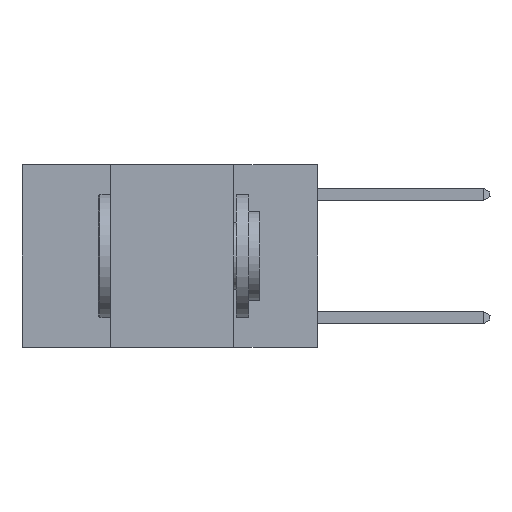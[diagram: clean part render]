
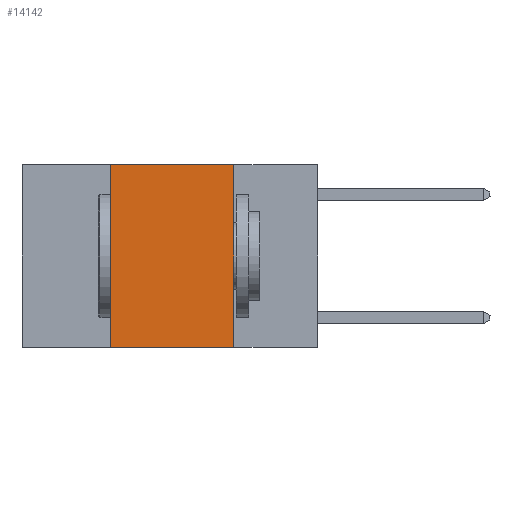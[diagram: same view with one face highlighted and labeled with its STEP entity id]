
A CAD part, left-side view. The second image highlights one B-rep face of the part: STEP entity #14142.
In plain terms, the highlighted planar face has unit normal (-1, 0, 0).
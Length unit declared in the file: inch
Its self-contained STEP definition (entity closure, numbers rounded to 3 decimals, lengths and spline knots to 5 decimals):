
#490 = CARTESIAN_POINT ( 'NONE',  ( 0., 0.42, 0. ) ) ;
#889 = VERTEX_POINT ( 'NONE', #3134 ) ;
#1014 = DIRECTION ( 'NONE',  ( 0., 0., -1. ) ) ;
#1304 = AXIS2_PLACEMENT_3D ( 'NONE', #6253, #11634, #16788 ) ;
#2366 = VECTOR ( 'NONE', #3803, 39.37008 ) ;
#2592 = CARTESIAN_POINT ( 'NONE',  ( 0., 0.17, -0.37 ) ) ;
#3063 = EDGE_CURVE ( 'NONE', #889, #5286, #8931, .T. ) ;
#3134 = CARTESIAN_POINT ( 'NONE',  ( 0., 0.42, -0.37 ) ) ;
#3528 = FACE_OUTER_BOUND ( 'NONE', #11966, .T. ) ;
#3563 = EDGE_CURVE ( 'NONE', #17010, #5286, #16999, .T. ) ;
#3803 = DIRECTION ( 'NONE',  ( 0., 0., 1. ) ) ;
#4730 = ORIENTED_EDGE ( 'NONE', *, *, #12457, .F. ) ;
#5286 = VERTEX_POINT ( 'NONE', #2592 ) ;
#6253 = CARTESIAN_POINT ( 'NONE',  ( 0., 0.6, 0. ) ) ;
#6334 = PLANE ( 'NONE',  #1304 ) ;
#7236 = CARTESIAN_POINT ( 'NONE',  ( 0., 0.6, 0. ) ) ;
#8492 = ORIENTED_EDGE ( 'NONE', *, *, #3563, .F. ) ;
#8548 = VECTOR ( 'NONE', #1014, 39.37008 ) ;
#8577 = ORIENTED_EDGE ( 'NONE', *, *, #12518, .F. ) ;
#8809 = VECTOR ( 'NONE', #13661, 39.37008 ) ;
#8931 = LINE ( 'NONE', #14211, #15452 ) ;
#11486 = LINE ( 'NONE', #16720, #2366 ) ;
#11634 = DIRECTION ( 'NONE',  ( 1., 0., 0. ) ) ;
#11966 = EDGE_LOOP ( 'NONE', ( #8492, #4730, #8577, #14532 ) ) ;
#12457 = EDGE_CURVE ( 'NONE', #17189, #17010, #16284, .T. ) ;
#12518 = EDGE_CURVE ( 'NONE', #889, #17189, #11486, .T. ) ;
#13661 = DIRECTION ( 'NONE',  ( 0., -1., 0. ) ) ;
#13683 = CARTESIAN_POINT ( 'NONE',  ( 0., 0.17, 0. ) ) ;
#14142 = ADVANCED_FACE ( 'NONE', ( #3528 ), #6334, .F. ) ;
#14211 = CARTESIAN_POINT ( 'NONE',  ( 0., 0.6, -0.37 ) ) ;
#14532 = ORIENTED_EDGE ( 'NONE', *, *, #3063, .T. ) ;
#15434 = DIRECTION ( 'NONE',  ( 0., -1., 0. ) ) ;
#15452 = VECTOR ( 'NONE', #15434, 39.37008 ) ;
#16284 = LINE ( 'NONE', #7236, #8809 ) ;
#16720 = CARTESIAN_POINT ( 'NONE',  ( 0., 0.42, 0. ) ) ;
#16788 = DIRECTION ( 'NONE',  ( 0., 0., -1. ) ) ;
#16909 = CARTESIAN_POINT ( 'NONE',  ( 0., 0.17, 0. ) ) ;
#16999 = LINE ( 'NONE', #16909, #8548 ) ;
#17010 = VERTEX_POINT ( 'NONE', #13683 ) ;
#17189 = VERTEX_POINT ( 'NONE', #490 ) ;
